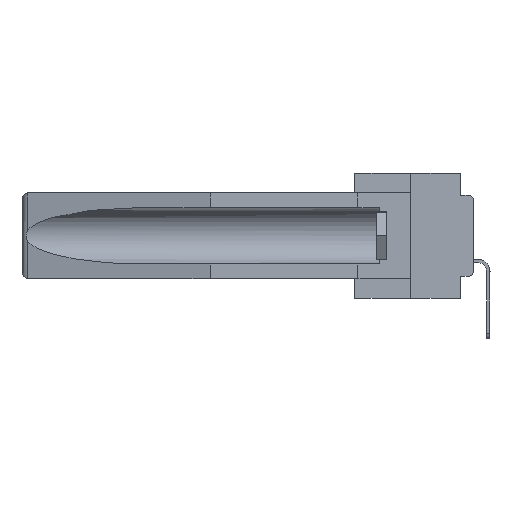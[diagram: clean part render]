
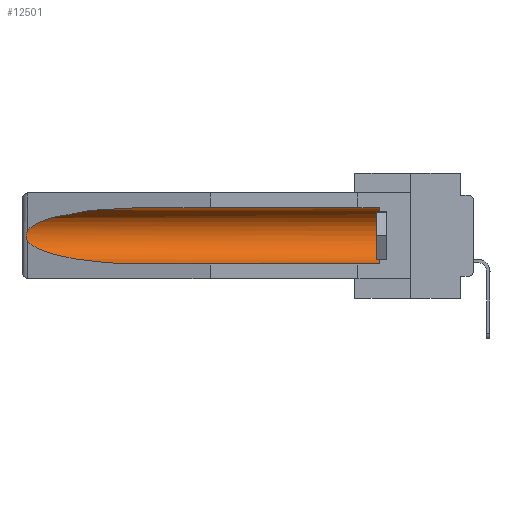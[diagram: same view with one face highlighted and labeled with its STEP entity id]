
A CAD part, left-side view. The second image highlights one B-rep face of the part: STEP entity #12501.
In plain terms, the highlighted cylindrical face has radius 2.857 mm (diameter 5.715 mm), a partial arc.
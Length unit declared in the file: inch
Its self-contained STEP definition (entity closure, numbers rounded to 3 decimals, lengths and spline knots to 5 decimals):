
#313 = CARTESIAN_POINT ( 'NONE',  ( 0.2673, 1.53269, -0.17917 ) ) ;
#366 = CARTESIAN_POINT ( 'NONE',  ( 0.26537, 1.52718, -0.14972 ) ) ;
#1074 = ORIENTED_EDGE ( 'NONE', *, *, #30459, .T. ) ;
#1172 = CARTESIAN_POINT ( 'NONE',  ( 0.155, 0.126, -0.1715 ) ) ;
#1759 = LINE ( 'NONE', #4331, #2918 ) ;
#1899 = EDGE_CURVE ( 'NONE', #21432, #18587, #18360, .T. ) ;
#2699 = CYLINDRICAL_SURFACE ( 'NONE', #2706, 0.1125 ) ;
#2706 = AXIS2_PLACEMENT_3D ( 'NONE', #10988, #7848, #22536 ) ;
#2918 = VECTOR ( 'NONE', #32474, 39.37008 ) ;
#2988 = VECTOR ( 'NONE', #31656, 39.37008 ) ;
#3053 = EDGE_CURVE ( 'NONE', #21116, #21432, #14740, .T. ) ;
#3071 = CARTESIAN_POINT ( 'NONE',  ( 0.26597, 1.52961, -0.15275 ) ) ;
#3443 = CARTESIAN_POINT ( 'NONE',  ( 0.26654, 1.53092, -0.15636 ) ) ;
#4331 = CARTESIAN_POINT ( 'NONE',  ( 0.155, -0.30754, -0.284 ) ) ;
#5439 = CARTESIAN_POINT ( 'NONE',  ( 0.21114, 1.30732, -0.059 ) ) ;
#6113 = CARTESIAN_POINT ( 'NONE',  ( 0.155, 0.126, -0.059 ) ) ;
#6149 = DIRECTION ( 'NONE',  ( 0., 0., 1. ) ) ;
#7848 = DIRECTION ( 'NONE',  ( 0., 1., 0. ) ) ;
#8580 = CARTESIAN_POINT ( 'NONE',  ( 0.25451, 1.48313, -0.24835 ) ) ;
#8628 = VERTEX_POINT ( 'NONE', #16360 ) ;
#9902 =( BOUNDED_CURVE ( )  B_SPLINE_CURVE ( 3, ( #22900, #8580, #33596, #11517 ),
 .UNSPECIFIED., .F., .F. ) 
 B_SPLINE_CURVE_WITH_KNOTS ( ( 4, 4 ),
 ( 0.1948, 1.5708 ),
 .UNSPECIFIED. ) 
 CURVE ( )  GEOMETRIC_REPRESENTATION_ITEM ( )  RATIONAL_B_SPLINE_CURVE ( ( 1., 0.848, 0.848, 1. ) ) 
 REPRESENTATION_ITEM ( '' )  );
#10316 = CIRCLE ( 'NONE', #17928, 0.1125 ) ;
#10988 = CARTESIAN_POINT ( 'NONE',  ( 0.155, -0.30754, -0.1715 ) ) ;
#11517 = CARTESIAN_POINT ( 'NONE',  ( 0.155, 1.07973, -0.284 ) ) ;
#11897 = CARTESIAN_POINT ( 'NONE',  ( 0.2673, 1.5327, -0.16383 ) ) ;
#12398 = EDGE_LOOP ( 'NONE', ( #13371, #18303, #1074, #33070, #23732, #35520 ) ) ;
#12404 = DIRECTION ( 'NONE',  ( 0., -1., 0. ) ) ;
#12501 = ADVANCED_FACE ( 'NONE', ( #28067 ), #2699, .F. ) ;
#13371 = ORIENTED_EDGE ( 'NONE', *, *, #1899, .T. ) ;
#13521 = VERTEX_POINT ( 'NONE', #18893 ) ;
#14304 = CARTESIAN_POINT ( 'NONE',  ( 0.2675, 1.53308, -0.16763 ) ) ;
#14497 = CARTESIAN_POINT ( 'NONE',  ( 0.26537, 1.52718, -0.19328 ) ) ;
#14740 = LINE ( 'NONE', #23167, #2988 ) ;
#16301 = CARTESIAN_POINT ( 'NONE',  ( 0.155, 1.07973, -0.059 ) ) ;
#16360 = CARTESIAN_POINT ( 'NONE',  ( 0.155, 0.126, -0.284 ) ) ;
#17887 = VERTEX_POINT ( 'NONE', #34880 ) ;
#17928 = AXIS2_PLACEMENT_3D ( 'NONE', #1172, #12404, #6149 ) ;
#18303 = ORIENTED_EDGE ( 'NONE', *, *, #18953, .T. ) ;
#18360 =( BOUNDED_CURVE ( )  B_SPLINE_CURVE ( 3, ( #16301, #5439, #18849, #27515 ),
 .UNSPECIFIED., .F., .F. ) 
 B_SPLINE_CURVE_WITH_KNOTS ( ( 4, 4 ),
 ( 4.71239, 6.08839 ),
 .UNSPECIFIED. ) 
 CURVE ( )  GEOMETRIC_REPRESENTATION_ITEM ( )  RATIONAL_B_SPLINE_CURVE ( ( 1., 0.848, 0.848, 1. ) ) 
 REPRESENTATION_ITEM ( '' )  );
#18587 = VERTEX_POINT ( 'NONE', #366 ) ;
#18849 = CARTESIAN_POINT ( 'NONE',  ( 0.25451, 1.48313, -0.09465 ) ) ;
#18893 = CARTESIAN_POINT ( 'NONE',  ( 0.155, 1.07973, -0.284 ) ) ;
#18953 = EDGE_CURVE ( 'NONE', #18587, #17887, #23390, .T. ) ;
#20150 = CARTESIAN_POINT ( 'NONE',  ( 0.2675, 1.53308, -0.17534 ) ) ;
#20348 = CARTESIAN_POINT ( 'NONE',  ( 0.26655, 1.53094, -0.18657 ) ) ;
#20392 = CARTESIAN_POINT ( 'NONE',  ( 0.155, 1.07973, -0.059 ) ) ;
#21116 = VERTEX_POINT ( 'NONE', #6113 ) ;
#21432 = VERTEX_POINT ( 'NONE', #20392 ) ;
#22536 = DIRECTION ( 'NONE',  ( 0., 0., 1. ) ) ;
#22745 = CARTESIAN_POINT ( 'NONE',  ( 0.26597, 1.5296, -0.19026 ) ) ;
#22900 = CARTESIAN_POINT ( 'NONE',  ( 0.26537, 1.52718, -0.19328 ) ) ;
#23167 = CARTESIAN_POINT ( 'NONE',  ( 0.155, -0.30754, -0.059 ) ) ;
#23390 = B_SPLINE_CURVE_WITH_KNOTS ( 'NONE', 3,
 ( #34158, #3071, #3443, #11897, #14304, #20150, #313, #20348, #22745, #14497 ),
 .UNSPECIFIED., .F., .F.,
 ( 4, 2, 2, 2, 4 ),
 ( 0., 0.00029, 0.00058, 0.00087, 0.00117 ),
 .UNSPECIFIED. ) ;
#23732 = ORIENTED_EDGE ( 'NONE', *, *, #28930, .T. ) ;
#27515 = CARTESIAN_POINT ( 'NONE',  ( 0.26537, 1.52718, -0.14972 ) ) ;
#28067 = FACE_OUTER_BOUND ( 'NONE', #12398, .T. ) ;
#28930 = EDGE_CURVE ( 'NONE', #8628, #21116, #10316, .T. ) ;
#30459 = EDGE_CURVE ( 'NONE', #17887, #13521, #9902, .T. ) ;
#31656 = DIRECTION ( 'NONE',  ( 0., 1., 0. ) ) ;
#32474 = DIRECTION ( 'NONE',  ( 0., 1., 0. ) ) ;
#33070 = ORIENTED_EDGE ( 'NONE', *, *, #33682, .F. ) ;
#33596 = CARTESIAN_POINT ( 'NONE',  ( 0.21114, 1.30732, -0.284 ) ) ;
#33682 = EDGE_CURVE ( 'NONE', #8628, #13521, #1759, .T. ) ;
#34158 = CARTESIAN_POINT ( 'NONE',  ( 0.26537, 1.52718, -0.14972 ) ) ;
#34880 = CARTESIAN_POINT ( 'NONE',  ( 0.26537, 1.52718, -0.19328 ) ) ;
#35520 = ORIENTED_EDGE ( 'NONE', *, *, #3053, .T. ) ;
